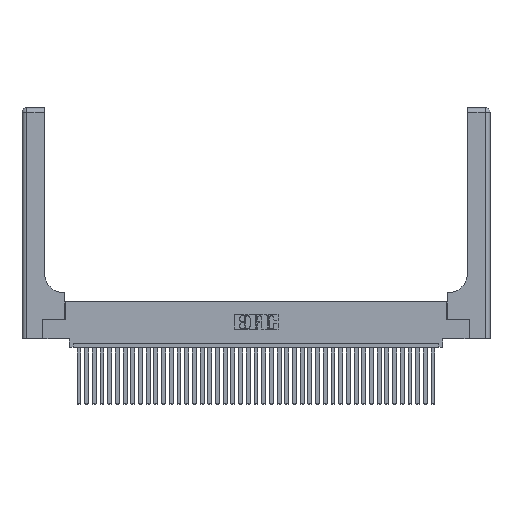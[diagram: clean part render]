
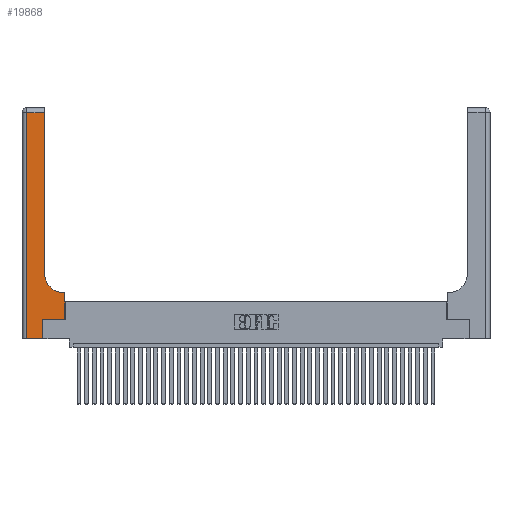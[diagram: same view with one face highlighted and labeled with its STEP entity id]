
A CAD part, top view. The second image highlights one B-rep face of the part: STEP entity #19868.
In plain terms, the highlighted planar face has unit normal (0, 0, 1).
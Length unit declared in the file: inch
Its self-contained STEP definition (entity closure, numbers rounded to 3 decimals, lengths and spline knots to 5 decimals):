
#972 = LINE ( 'NONE', #5288, #28883 ) ;
#1725 = VECTOR ( 'NONE', #10343, 39.37008 ) ;
#2563 = CARTESIAN_POINT ( 'NONE',  ( 0.06, 2.94, 0.37 ) ) ;
#3012 = EDGE_CURVE ( 'NONE', #14239, #14969, #18525, .T. ) ;
#3080 = LINE ( 'NONE', #25238, #28614 ) ;
#3413 = DIRECTION ( 'NONE',  ( -1., 0., 0. ) ) ;
#3681 = PLANE ( 'NONE',  #17585 ) ;
#3763 = DIRECTION ( 'NONE',  ( 1., 0., 0. ) ) ;
#4307 = EDGE_LOOP ( 'NONE', ( #27910, #26454, #7517, #13905, #21660, #18340, #14984, #7296, #6326 ) ) ;
#4582 = CARTESIAN_POINT ( 'NONE',  ( 0.5415, 0.6, 0.37 ) ) ;
#4758 = CARTESIAN_POINT ( 'NONE',  ( 0.269, 0.25, 0.37 ) ) ;
#5288 = CARTESIAN_POINT ( 'NONE',  ( 0.06, 3., 0.37 ) ) ;
#6326 = ORIENTED_EDGE ( 'NONE', *, *, #16760, .T. ) ;
#6363 = LINE ( 'NONE', #10161, #18430 ) ;
#6482 = CARTESIAN_POINT ( 'NONE',  ( 0., 3., 0.37 ) ) ;
#7296 = ORIENTED_EDGE ( 'NONE', *, *, #13556, .T. ) ;
#7481 = VECTOR ( 'NONE', #13716, 39.37008 ) ;
#7517 = ORIENTED_EDGE ( 'NONE', *, *, #8389, .T. ) ;
#8389 = EDGE_CURVE ( 'NONE', #39429, #14328, #972, .T. ) ;
#8668 = CARTESIAN_POINT ( 'NONE',  ( 0.2915, 2.94, 0.37 ) ) ;
#9591 = VERTEX_POINT ( 'NONE', #28717 ) ;
#10161 = CARTESIAN_POINT ( 'NONE',  ( 0., 0., 0.37 ) ) ;
#10343 = DIRECTION ( 'NONE',  ( 0., 1., 0. ) ) ;
#11335 = LINE ( 'NONE', #25690, #1725 ) ;
#11560 = EDGE_CURVE ( 'NONE', #9591, #14239, #3080, .T. ) ;
#11729 = CARTESIAN_POINT ( 'NONE',  ( 0.2915, 0.6, 0.37 ) ) ;
#12260 = LINE ( 'NONE', #31200, #30097 ) ;
#12543 = FACE_OUTER_BOUND ( 'NONE', #4307, .T. ) ;
#12745 = DIRECTION ( 'NONE',  ( 0., 1., 0. ) ) ;
#13556 = EDGE_CURVE ( 'NONE', #35718, #31864, #35811, .T. ) ;
#13716 = DIRECTION ( 'NONE',  ( 0., 1., 0. ) ) ;
#13905 = ORIENTED_EDGE ( 'NONE', *, *, #27614, .T. ) ;
#14219 = AXIS2_PLACEMENT_3D ( 'NONE', #24627, #17918, #3763 ) ;
#14239 = VERTEX_POINT ( 'NONE', #22634 ) ;
#14328 = VERTEX_POINT ( 'NONE', #29766 ) ;
#14787 = LINE ( 'NONE', #28362, #7481 ) ;
#14969 = VERTEX_POINT ( 'NONE', #39856 ) ;
#14984 = ORIENTED_EDGE ( 'NONE', *, *, #26497, .T. ) ;
#15681 = DIRECTION ( 'NONE',  ( 0., 0., -1. ) ) ;
#16645 = DIRECTION ( 'NONE',  ( 1., 0., 0. ) ) ;
#16760 = EDGE_CURVE ( 'NONE', #31864, #32514, #28842, .T. ) ;
#17585 = AXIS2_PLACEMENT_3D ( 'NONE', #6482, #15681, #3413 ) ;
#17918 = DIRECTION ( 'NONE',  ( 0., 0., -1. ) ) ;
#17976 = VECTOR ( 'NONE', #26936, 39.37008 ) ;
#18340 = ORIENTED_EDGE ( 'NONE', *, *, #3012, .T. ) ;
#18430 = VECTOR ( 'NONE', #16645, 39.37008 ) ;
#18525 = LINE ( 'NONE', #4758, #24350 ) ;
#19868 = ADVANCED_FACE ( 'NONE', ( #12543 ), #3681, .F. ) ;
#21660 = ORIENTED_EDGE ( 'NONE', *, *, #11560, .T. ) ;
#22053 = DIRECTION ( 'NONE',  ( -1., 0., 0. ) ) ;
#22634 = CARTESIAN_POINT ( 'NONE',  ( 0.269, 0.25, 0.37 ) ) ;
#23695 = CARTESIAN_POINT ( 'NONE',  ( 0.5585, 0.6, 0.37 ) ) ;
#24350 = VECTOR ( 'NONE', #26265, 39.37008 ) ;
#24627 = CARTESIAN_POINT ( 'NONE',  ( 0.5415, 0.85, 0.37 ) ) ;
#25238 = CARTESIAN_POINT ( 'NONE',  ( 0.269, 0., 0.37 ) ) ;
#25690 = CARTESIAN_POINT ( 'NONE',  ( 0.5585, 0.25, 0.37 ) ) ;
#26175 = EDGE_CURVE ( 'NONE', #32514, #35323, #14787, .T. ) ;
#26265 = DIRECTION ( 'NONE',  ( 1., 0., 0. ) ) ;
#26454 = ORIENTED_EDGE ( 'NONE', *, *, #26815, .T. ) ;
#26497 = EDGE_CURVE ( 'NONE', #14969, #35718, #11335, .T. ) ;
#26812 = DIRECTION ( 'NONE',  ( 0., -1., 0. ) ) ;
#26815 = EDGE_CURVE ( 'NONE', #35323, #39429, #12260, .T. ) ;
#26936 = DIRECTION ( 'NONE',  ( -1., 0., 0. ) ) ;
#27614 = EDGE_CURVE ( 'NONE', #14328, #9591, #6363, .T. ) ;
#27910 = ORIENTED_EDGE ( 'NONE', *, *, #26175, .T. ) ;
#28362 = CARTESIAN_POINT ( 'NONE',  ( 0.2915, 3., 0.37 ) ) ;
#28614 = VECTOR ( 'NONE', #12745, 39.37008 ) ;
#28717 = CARTESIAN_POINT ( 'NONE',  ( 0.269, 0., 0.37 ) ) ;
#28842 = CIRCLE ( 'NONE', #14219, 0.25 ) ;
#28883 = VECTOR ( 'NONE', #26812, 39.37008 ) ;
#29766 = CARTESIAN_POINT ( 'NONE',  ( 0.06, 0., 0.37 ) ) ;
#30097 = VECTOR ( 'NONE', #22053, 39.37008 ) ;
#30854 = CARTESIAN_POINT ( 'NONE',  ( 0.2915, 0.85, 0.37 ) ) ;
#31200 = CARTESIAN_POINT ( 'NONE',  ( 0., 2.94, 0.37 ) ) ;
#31864 = VERTEX_POINT ( 'NONE', #4582 ) ;
#32514 = VERTEX_POINT ( 'NONE', #30854 ) ;
#35323 = VERTEX_POINT ( 'NONE', #8668 ) ;
#35718 = VERTEX_POINT ( 'NONE', #23695 ) ;
#35811 = LINE ( 'NONE', #11729, #17976 ) ;
#39429 = VERTEX_POINT ( 'NONE', #2563 ) ;
#39856 = CARTESIAN_POINT ( 'NONE',  ( 0.5585, 0.25, 0.37 ) ) ;
